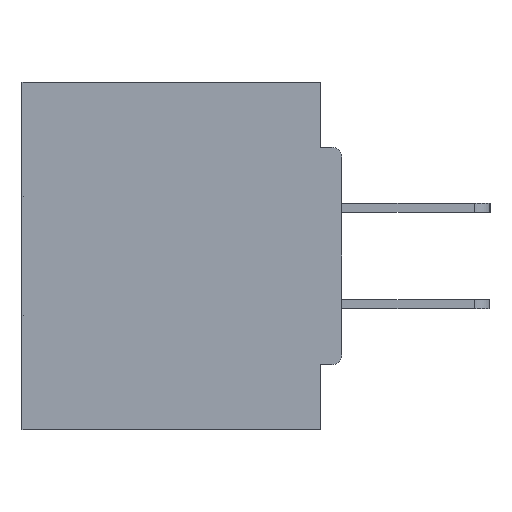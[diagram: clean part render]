
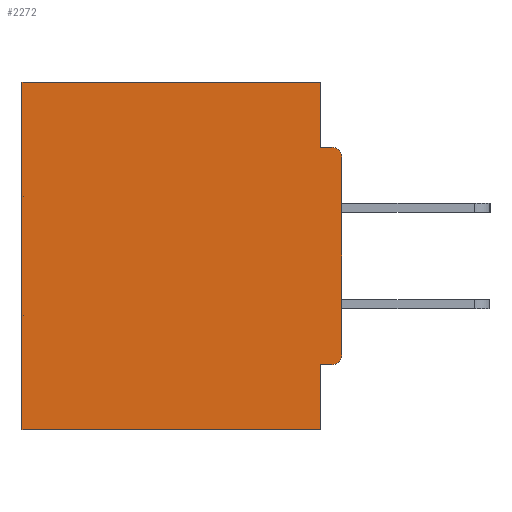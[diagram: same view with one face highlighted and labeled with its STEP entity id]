
A CAD part, left-side view. The second image highlights one B-rep face of the part: STEP entity #2272.
In plain terms, the highlighted planar face has unit normal (-1, 0, 0).
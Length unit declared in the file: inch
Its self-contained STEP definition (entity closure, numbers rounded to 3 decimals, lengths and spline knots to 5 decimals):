
#13 = CARTESIAN_POINT ( 'NONE',  ( 0.298, 0.031, -0.5 ) ) ;
#361 = LINE ( 'NONE', #29795, #33504 ) ;
#1138 = VECTOR ( 'NONE', #18994, 39.37008 ) ;
#1213 = VERTEX_POINT ( 'NONE', #30411 ) ;
#1762 = DIRECTION ( 'NONE',  ( 0., 0., -1. ) ) ;
#2272 = ADVANCED_FACE ( 'NONE', ( #10978 ), #8077, .F. ) ;
#3021 = VERTEX_POINT ( 'NONE', #36396 ) ;
#3646 = EDGE_CURVE ( 'NONE', #27671, #27036, #19450, .T. ) ;
#3925 = CARTESIAN_POINT ( 'NONE',  ( 0.298, 0., -0.1085 ) ) ;
#3955 = ORIENTED_EDGE ( 'NONE', *, *, #7415, .T. ) ;
#4718 = LINE ( 'NONE', #15742, #1138 ) ;
#4861 = VERTEX_POINT ( 'NONE', #6621 ) ;
#5011 = CIRCLE ( 'NONE', #26845, 0.015 ) ;
#5113 = CARTESIAN_POINT ( 'NONE',  ( 0.298, 0., 0. ) ) ;
#6078 = ORIENTED_EDGE ( 'NONE', *, *, #16283, .F. ) ;
#6250 = LINE ( 'NONE', #14782, #38785 ) ;
#6621 = CARTESIAN_POINT ( 'NONE',  ( 0.298, 0.015, -0.0935 ) ) ;
#7076 = CARTESIAN_POINT ( 'NONE',  ( 0.298, 0.031, -0.5 ) ) ;
#7331 = CARTESIAN_POINT ( 'NONE',  ( 0.298, 0., -0.5 ) ) ;
#7415 = EDGE_CURVE ( 'NONE', #15929, #4861, #5011, .T. ) ;
#7589 = ORIENTED_EDGE ( 'NONE', *, *, #28132, .F. ) ;
#7639 = EDGE_CURVE ( 'NONE', #1213, #19116, #41164, .T. ) ;
#8077 = PLANE ( 'NONE',  #14993 ) ;
#8959 = ORIENTED_EDGE ( 'NONE', *, *, #12287, .T. ) ;
#9300 = VECTOR ( 'NONE', #40039, 39.37008 ) ;
#9486 = LINE ( 'NONE', #26842, #19164 ) ;
#9554 = CARTESIAN_POINT ( 'NONE',  ( 0.298, 0.015, -0.1085 ) ) ;
#10045 = CARTESIAN_POINT ( 'NONE',  ( 0.298, 0.031, -0.4065 ) ) ;
#10046 = VERTEX_POINT ( 'NONE', #14930 ) ;
#10081 = ORIENTED_EDGE ( 'NONE', *, *, #7639, .T. ) ;
#10270 = DIRECTION ( 'NONE',  ( 0., 1., 0. ) ) ;
#10978 = FACE_OUTER_BOUND ( 'NONE', #16882, .T. ) ;
#11049 = DIRECTION ( 'NONE',  ( 0., 1., 0. ) ) ;
#11782 = CARTESIAN_POINT ( 'NONE',  ( 0.298, 0., 0. ) ) ;
#12176 = ORIENTED_EDGE ( 'NONE', *, *, #40667, .T. ) ;
#12287 = EDGE_CURVE ( 'NONE', #3021, #31952, #30898, .T. ) ;
#12822 = DIRECTION ( 'NONE',  ( -1., 0., 0. ) ) ;
#13357 = VECTOR ( 'NONE', #11049, 39.37008 ) ;
#14782 = CARTESIAN_POINT ( 'NONE',  ( 0.298, 0., 0. ) ) ;
#14930 = CARTESIAN_POINT ( 'NONE',  ( 0.298, 0.031, 0. ) ) ;
#14993 = AXIS2_PLACEMENT_3D ( 'NONE', #11782, #24925, #34545 ) ;
#15742 = CARTESIAN_POINT ( 'NONE',  ( 0.298, 0.031, -0.5 ) ) ;
#15929 = VERTEX_POINT ( 'NONE', #3925 ) ;
#16283 = EDGE_CURVE ( 'NONE', #27036, #19116, #34205, .T. ) ;
#16882 = EDGE_LOOP ( 'NONE', ( #3955, #31413, #27007, #12176, #10081, #6078, #38094, #7589, #8959, #23002 ) ) ;
#17840 = DIRECTION ( 'NONE',  ( 0., 1., 0. ) ) ;
#18994 = DIRECTION ( 'NONE',  ( 0., 0., -1. ) ) ;
#19116 = VERTEX_POINT ( 'NONE', #24663 ) ;
#19164 = VECTOR ( 'NONE', #36624, 39.37008 ) ;
#19450 = LINE ( 'NONE', #13, #9300 ) ;
#21099 = CARTESIAN_POINT ( 'NONE',  ( 0.298, 0.015, -0.3915 ) ) ;
#21399 = DIRECTION ( 'NONE',  ( 0., 0., -1. ) ) ;
#22027 = EDGE_CURVE ( 'NONE', #10046, #27384, #4718, .T. ) ;
#23002 = ORIENTED_EDGE ( 'NONE', *, *, #31268, .F. ) ;
#24663 = CARTESIAN_POINT ( 'NONE',  ( 0.298, 0.46, -0.5 ) ) ;
#24925 = DIRECTION ( 'NONE',  ( 1., 0., 0. ) ) ;
#26842 = CARTESIAN_POINT ( 'NONE',  ( 0.298, 0., -0.0935 ) ) ;
#26845 = AXIS2_PLACEMENT_3D ( 'NONE', #9554, #12822, #35559 ) ;
#27007 = ORIENTED_EDGE ( 'NONE', *, *, #22027, .F. ) ;
#27036 = VERTEX_POINT ( 'NONE', #7076 ) ;
#27384 = VERTEX_POINT ( 'NONE', #34975 ) ;
#27649 = DIRECTION ( 'NONE',  ( -1., 0., 0. ) ) ;
#27671 = VERTEX_POINT ( 'NONE', #10045 ) ;
#28132 = EDGE_CURVE ( 'NONE', #3021, #27671, #361, .T. ) ;
#28954 = CARTESIAN_POINT ( 'NONE',  ( 0.298, 0., -0.3915 ) ) ;
#29795 = CARTESIAN_POINT ( 'NONE',  ( 0.298, 0., -0.4065 ) ) ;
#30411 = CARTESIAN_POINT ( 'NONE',  ( 0.298, 0.46, 0. ) ) ;
#30898 = CIRCLE ( 'NONE', #38358, 0.015 ) ;
#31268 = EDGE_CURVE ( 'NONE', #15929, #31952, #6250, .T. ) ;
#31400 = VECTOR ( 'NONE', #17840, 39.37008 ) ;
#31413 = ORIENTED_EDGE ( 'NONE', *, *, #39859, .F. ) ;
#31952 = VERTEX_POINT ( 'NONE', #28954 ) ;
#33504 = VECTOR ( 'NONE', #10270, 39.37008 ) ;
#34205 = LINE ( 'NONE', #7331, #13357 ) ;
#34545 = DIRECTION ( 'NONE',  ( 0., 0., -1. ) ) ;
#34975 = CARTESIAN_POINT ( 'NONE',  ( 0.298, 0.031, -0.0935 ) ) ;
#35057 = VECTOR ( 'NONE', #21399, 39.37008 ) ;
#35559 = DIRECTION ( 'NONE',  ( 0., 0., -1. ) ) ;
#36396 = CARTESIAN_POINT ( 'NONE',  ( 0.298, 0.015, -0.4065 ) ) ;
#36624 = DIRECTION ( 'NONE',  ( 0., -1., 0. ) ) ;
#37570 = DIRECTION ( 'NONE',  ( 0., 0., -1. ) ) ;
#37578 = CARTESIAN_POINT ( 'NONE',  ( 0.298, 0.46, 0. ) ) ;
#38094 = ORIENTED_EDGE ( 'NONE', *, *, #3646, .F. ) ;
#38358 = AXIS2_PLACEMENT_3D ( 'NONE', #21099, #27649, #37570 ) ;
#38785 = VECTOR ( 'NONE', #1762, 39.37008 ) ;
#39859 = EDGE_CURVE ( 'NONE', #27384, #4861, #9486, .T. ) ;
#39974 = LINE ( 'NONE', #5113, #31400 ) ;
#40039 = DIRECTION ( 'NONE',  ( 0., 0., -1. ) ) ;
#40667 = EDGE_CURVE ( 'NONE', #10046, #1213, #39974, .T. ) ;
#41164 = LINE ( 'NONE', #37578, #35057 ) ;
